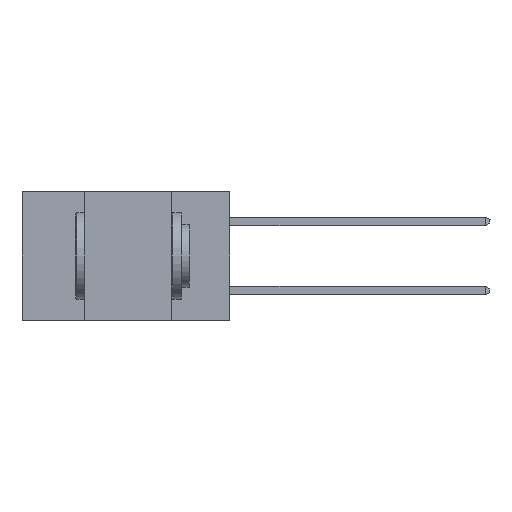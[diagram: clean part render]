
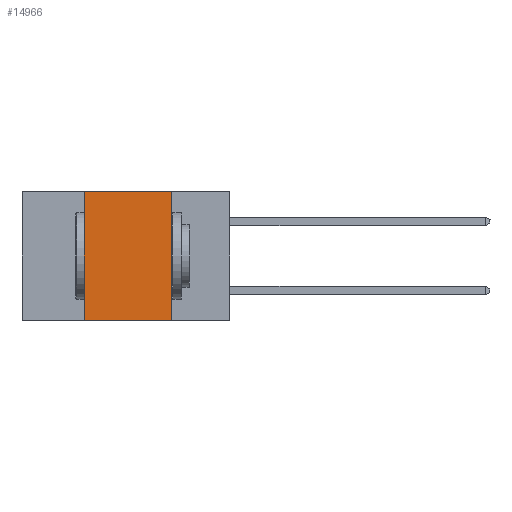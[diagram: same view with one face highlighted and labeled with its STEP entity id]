
A CAD part, left-side view. The second image highlights one B-rep face of the part: STEP entity #14966.
In plain terms, the highlighted planar face has unit normal (-1, 0, 0).
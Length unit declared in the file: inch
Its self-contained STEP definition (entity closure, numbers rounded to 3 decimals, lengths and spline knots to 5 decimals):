
#259 = DIRECTION ( 'NONE',  ( 0., 0., 1. ) ) ;
#1249 = EDGE_LOOP ( 'NONE', ( #16846, #7513, #5143, #10792 ) ) ;
#1440 = EDGE_CURVE ( 'NONE', #9846, #16360, #9929, .T. ) ;
#3240 = CARTESIAN_POINT ( 'NONE',  ( 0., 0.6, 0. ) ) ;
#4125 = VECTOR ( 'NONE', #15727, 39.37008 ) ;
#4225 = CARTESIAN_POINT ( 'NONE',  ( 0., 0.17, -0.37 ) ) ;
#4601 = FACE_OUTER_BOUND ( 'NONE', #1249, .T. ) ;
#4881 = CARTESIAN_POINT ( 'NONE',  ( 0., 0.17, 0. ) ) ;
#5143 = ORIENTED_EDGE ( 'NONE', *, *, #1440, .F. ) ;
#7150 = CARTESIAN_POINT ( 'NONE',  ( 0., 0.42, -0.37 ) ) ;
#7513 = ORIENTED_EDGE ( 'NONE', *, *, #15769, .F. ) ;
#7772 = AXIS2_PLACEMENT_3D ( 'NONE', #3240, #15875, #20855 ) ;
#8057 = CARTESIAN_POINT ( 'NONE',  ( 0., 0.17, -0.37 ) ) ;
#8433 = VERTEX_POINT ( 'NONE', #4225 ) ;
#9373 = PLANE ( 'NONE',  #7772 ) ;
#9846 = VERTEX_POINT ( 'NONE', #13341 ) ;
#9929 = LINE ( 'NONE', #7150, #16733 ) ;
#10792 = ORIENTED_EDGE ( 'NONE', *, *, #17168, .T. ) ;
#11575 = VECTOR ( 'NONE', #14221, 39.37008 ) ;
#12324 = VECTOR ( 'NONE', #17758, 39.37008 ) ;
#12521 = LINE ( 'NONE', #20595, #4125 ) ;
#13341 = CARTESIAN_POINT ( 'NONE',  ( 0., 0.42, -0.37 ) ) ;
#14221 = DIRECTION ( 'NONE',  ( 0., -1., 0. ) ) ;
#14966 = ADVANCED_FACE ( 'NONE', ( #4601 ), #9373, .F. ) ;
#15727 = DIRECTION ( 'NONE',  ( 0., -1., 0. ) ) ;
#15769 = EDGE_CURVE ( 'NONE', #16360, #19622, #20701, .T. ) ;
#15875 = DIRECTION ( 'NONE',  ( 1., 0., 0. ) ) ;
#16360 = VERTEX_POINT ( 'NONE', #20865 ) ;
#16733 = VECTOR ( 'NONE', #259, 39.37008 ) ;
#16846 = ORIENTED_EDGE ( 'NONE', *, *, #19220, .F. ) ;
#17168 = EDGE_CURVE ( 'NONE', #9846, #8433, #12521, .T. ) ;
#17737 = CARTESIAN_POINT ( 'NONE',  ( 0., 0.6, 0. ) ) ;
#17758 = DIRECTION ( 'NONE',  ( 0., 0., -1. ) ) ;
#19220 = EDGE_CURVE ( 'NONE', #19622, #8433, #19456, .T. ) ;
#19456 = LINE ( 'NONE', #8057, #12324 ) ;
#19622 = VERTEX_POINT ( 'NONE', #4881 ) ;
#20595 = CARTESIAN_POINT ( 'NONE',  ( 0., 0.6, -0.37 ) ) ;
#20701 = LINE ( 'NONE', #17737, #11575 ) ;
#20855 = DIRECTION ( 'NONE',  ( 0., 0., -1. ) ) ;
#20865 = CARTESIAN_POINT ( 'NONE',  ( 0., 0.42, 0. ) ) ;
